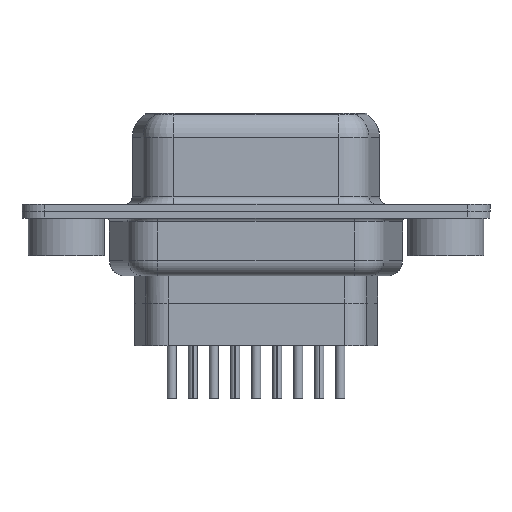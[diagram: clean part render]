
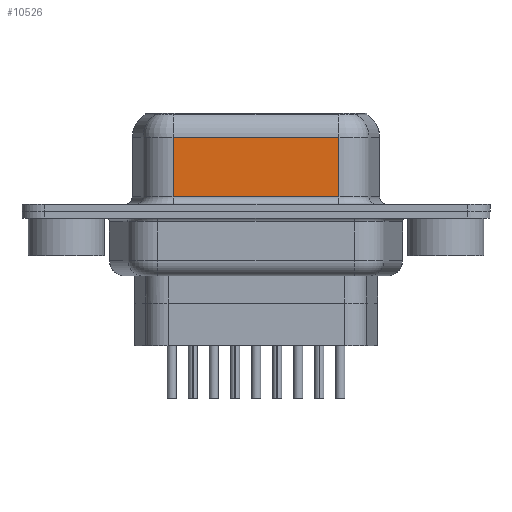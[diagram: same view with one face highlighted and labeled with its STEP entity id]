
A CAD part, front view. The second image highlights one B-rep face of the part: STEP entity #10526.
In plain terms, the highlighted planar face has unit normal (0, -1, 0).
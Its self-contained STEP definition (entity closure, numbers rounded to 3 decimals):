
#942 = CARTESIAN_POINT ( 'NONE',  ( 17.957, -3.95, 4.85 ) ) ;
#1053 = VERTEX_POINT ( 'NONE', #942 ) ;
#1112 = EDGE_CURVE ( 'NONE', #1053, #6725, #3700, .T. ) ;
#1458 = VECTOR ( 'NONE', #13550, 1000. ) ;
#1675 = ORIENTED_EDGE ( 'NONE', *, *, #15418, .T. ) ;
#2007 = AXIS2_PLACEMENT_3D ( 'NONE', #6959, #11899, #20813 ) ;
#2027 = CARTESIAN_POINT ( 'NONE',  ( 17.957, -3.95, 0.95 ) ) ;
#3322 = VERTEX_POINT ( 'NONE', #15684 ) ;
#3700 = LINE ( 'NONE', #17335, #19465 ) ;
#3712 = LINE ( 'NONE', #5653, #14089 ) ;
#5653 = CARTESIAN_POINT ( 'NONE',  ( 7.033, -3.95, 6.6 ) ) ;
#5888 = VERTEX_POINT ( 'NONE', #8953 ) ;
#6056 = LINE ( 'NONE', #21530, #12748 ) ;
#6725 = VERTEX_POINT ( 'NONE', #2027 ) ;
#6959 = CARTESIAN_POINT ( 'NONE',  ( 17.957, -3.95, 6.6 ) ) ;
#8953 = CARTESIAN_POINT ( 'NONE',  ( 7.033, -3.95, 4.85 ) ) ;
#9853 = ORIENTED_EDGE ( 'NONE', *, *, #20612, .T. ) ;
#10104 = EDGE_CURVE ( 'NONE', #5888, #3322, #3712, .T. ) ;
#10116 = ORIENTED_EDGE ( 'NONE', *, *, #1112, .F. ) ;
#10526 = ADVANCED_FACE ( 'NONE', ( #12016 ), #22537, .F. ) ;
#10708 = DIRECTION ( 'NONE',  ( 0., 0., -1. ) ) ;
#11899 = DIRECTION ( 'NONE',  ( 0., 1., 0. ) ) ;
#12016 = FACE_OUTER_BOUND ( 'NONE', #17307, .T. ) ;
#12748 = VECTOR ( 'NONE', #14681, 1000. ) ;
#13029 = ORIENTED_EDGE ( 'NONE', *, *, #10104, .T. ) ;
#13550 = DIRECTION ( 'NONE',  ( -1., 0., 0. ) ) ;
#13769 = CARTESIAN_POINT ( 'NONE',  ( 17.957, -3.95, 4.85 ) ) ;
#14089 = VECTOR ( 'NONE', #10708, 1000. ) ;
#14681 = DIRECTION ( 'NONE',  ( 1., 0., 0. ) ) ;
#15418 = EDGE_CURVE ( 'NONE', #1053, #5888, #15500, .T. ) ;
#15500 = LINE ( 'NONE', #13769, #1458 ) ;
#15684 = CARTESIAN_POINT ( 'NONE',  ( 7.033, -3.95, 0.95 ) ) ;
#17307 = EDGE_LOOP ( 'NONE', ( #10116, #1675, #13029, #9853 ) ) ;
#17335 = CARTESIAN_POINT ( 'NONE',  ( 17.957, -3.95, 6.6 ) ) ;
#19465 = VECTOR ( 'NONE', #20765, 1000. ) ;
#20612 = EDGE_CURVE ( 'NONE', #3322, #6725, #6056, .T. ) ;
#20765 = DIRECTION ( 'NONE',  ( 0., 0., -1. ) ) ;
#20813 = DIRECTION ( 'NONE',  ( 0., 0., 1. ) ) ;
#21530 = CARTESIAN_POINT ( 'NONE',  ( 17.957, -3.95, 0.95 ) ) ;
#22537 = PLANE ( 'NONE',  #2007 ) ;
